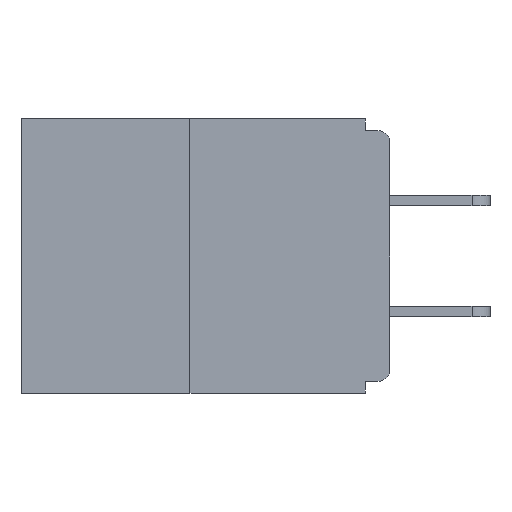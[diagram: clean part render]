
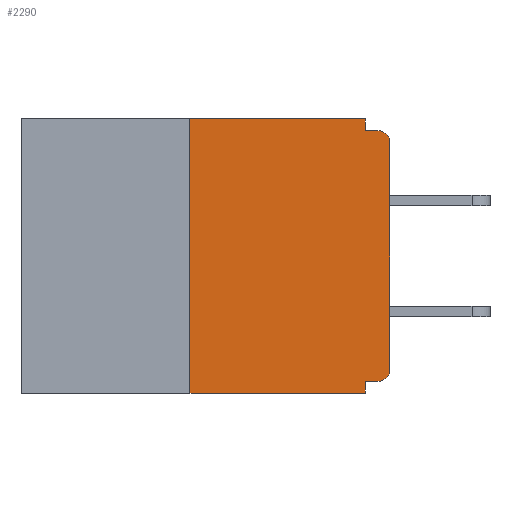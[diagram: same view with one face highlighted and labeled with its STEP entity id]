
A CAD part, left-side view. The second image highlights one B-rep face of the part: STEP entity #2290.
In plain terms, the highlighted planar face has unit normal (-1, 0, 0).
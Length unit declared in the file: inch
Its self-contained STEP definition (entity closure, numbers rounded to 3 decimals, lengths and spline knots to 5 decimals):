
#183 = PLANE ( 'NONE',  #4799 ) ;
#190 = VERTEX_POINT ( 'NONE', #14920 ) ;
#453 = ORIENTED_EDGE ( 'NONE', *, *, #7173, .F. ) ;
#699 = EDGE_CURVE ( 'NONE', #190, #17312, #8416, .T. ) ;
#786 = CARTESIAN_POINT ( 'NONE',  ( 0., 0., -0.03 ) ) ;
#973 = CARTESIAN_POINT ( 'NONE',  ( 0., 0.015, -0.328 ) ) ;
#1226 = VERTEX_POINT ( 'NONE', #10289 ) ;
#1649 = EDGE_CURVE ( 'NONE', #17980, #9314, #11730, .T. ) ;
#1697 = DIRECTION ( 'NONE',  ( 0., 0., -1. ) ) ;
#1724 = CARTESIAN_POINT ( 'NONE',  ( 0., 0., -0.015 ) ) ;
#2184 = CARTESIAN_POINT ( 'NONE',  ( 0., 0.015, -0.313 ) ) ;
#2290 = ADVANCED_FACE ( 'NONE', ( #3118 ), #183, .F. ) ;
#2786 = CARTESIAN_POINT ( 'NONE',  ( 0., 0.46, 0. ) ) ;
#2792 = LINE ( 'NONE', #15246, #10029 ) ;
#2833 = DIRECTION ( 'NONE',  ( 0., 0., 1. ) ) ;
#3118 = FACE_OUTER_BOUND ( 'NONE', #16494, .T. ) ;
#3314 = CARTESIAN_POINT ( 'NONE',  ( 0., 0.031, -0.328 ) ) ;
#3999 = CIRCLE ( 'NONE', #13432, 0.015 ) ;
#4441 = DIRECTION ( 'NONE',  ( 0., 0., -1. ) ) ;
#4478 = DIRECTION ( 'NONE',  ( 1., 0., 0. ) ) ;
#4491 = VERTEX_POINT ( 'NONE', #16919 ) ;
#4651 = EDGE_CURVE ( 'NONE', #17312, #1226, #11841, .T. ) ;
#4799 = AXIS2_PLACEMENT_3D ( 'NONE', #5992, #4478, #1697 ) ;
#4962 = DIRECTION ( 'NONE',  ( 0., 0., -1. ) ) ;
#5008 = ORIENTED_EDGE ( 'NONE', *, *, #4651, .F. ) ;
#5094 = DIRECTION ( 'NONE',  ( 0., 0., -1. ) ) ;
#5135 = CARTESIAN_POINT ( 'NONE',  ( 0., 0.46, -0.343 ) ) ;
#5992 = CARTESIAN_POINT ( 'NONE',  ( 0., 0.46, 0. ) ) ;
#6024 = DIRECTION ( 'NONE',  ( 0., -1., 0. ) ) ;
#7113 = VERTEX_POINT ( 'NONE', #15981 ) ;
#7124 = ORIENTED_EDGE ( 'NONE', *, *, #18024, .T. ) ;
#7173 = EDGE_CURVE ( 'NONE', #10045, #7966, #10859, .T. ) ;
#7211 = ORIENTED_EDGE ( 'NONE', *, *, #13579, .F. ) ;
#7966 = VERTEX_POINT ( 'NONE', #3314 ) ;
#8043 = VECTOR ( 'NONE', #14109, 39.37008 ) ;
#8416 = LINE ( 'NONE', #2786, #13779 ) ;
#8475 = ORIENTED_EDGE ( 'NONE', *, *, #1649, .T. ) ;
#8771 = VECTOR ( 'NONE', #2833, 39.37008 ) ;
#8884 = CARTESIAN_POINT ( 'NONE',  ( 0., 0.031, 0. ) ) ;
#9164 = CARTESIAN_POINT ( 'NONE',  ( 0., 0.015, -0.015 ) ) ;
#9314 = VERTEX_POINT ( 'NONE', #9164 ) ;
#9770 = EDGE_CURVE ( 'NONE', #1226, #9314, #11956, .T. ) ;
#9935 = DIRECTION ( 'NONE',  ( 0., -1., 0. ) ) ;
#10029 = VECTOR ( 'NONE', #5094, 39.37008 ) ;
#10038 = LINE ( 'NONE', #5135, #8043 ) ;
#10045 = VERTEX_POINT ( 'NONE', #973 ) ;
#10141 = VECTOR ( 'NONE', #13106, 39.37008 ) ;
#10289 = CARTESIAN_POINT ( 'NONE',  ( 0., 0.031, -0.015 ) ) ;
#10817 = DIRECTION ( 'NONE',  ( -1., 0., 0. ) ) ;
#10859 = LINE ( 'NONE', #15917, #11521 ) ;
#11047 = AXIS2_PLACEMENT_3D ( 'NONE', #14009, #10817, #4962 ) ;
#11521 = VECTOR ( 'NONE', #14372, 39.37008 ) ;
#11730 = CIRCLE ( 'NONE', #11047, 0.015 ) ;
#11841 = LINE ( 'NONE', #8884, #16958 ) ;
#11940 = LINE ( 'NONE', #14514, #10141 ) ;
#11956 = LINE ( 'NONE', #1724, #12179 ) ;
#12179 = VECTOR ( 'NONE', #6024, 39.37008 ) ;
#12334 = VERTEX_POINT ( 'NONE', #12442 ) ;
#12442 = CARTESIAN_POINT ( 'NONE',  ( 0., 0., -0.313 ) ) ;
#12531 = EDGE_CURVE ( 'NONE', #7113, #4491, #10038, .T. ) ;
#13106 = DIRECTION ( 'NONE',  ( 0., 0., 1. ) ) ;
#13432 = AXIS2_PLACEMENT_3D ( 'NONE', #2184, #17759, #13663 ) ;
#13579 = EDGE_CURVE ( 'NONE', #7966, #4491, #2792, .T. ) ;
#13663 = DIRECTION ( 'NONE',  ( 0., 0., -1. ) ) ;
#13665 = ORIENTED_EDGE ( 'NONE', *, *, #699, .F. ) ;
#13779 = VECTOR ( 'NONE', #9935, 39.37008 ) ;
#14009 = CARTESIAN_POINT ( 'NONE',  ( 0., 0.015, -0.03 ) ) ;
#14073 = ORIENTED_EDGE ( 'NONE', *, *, #17715, .F. ) ;
#14109 = DIRECTION ( 'NONE',  ( 0., -1., 0. ) ) ;
#14335 = LINE ( 'NONE', #17214, #8771 ) ;
#14372 = DIRECTION ( 'NONE',  ( 0., 1., 0. ) ) ;
#14514 = CARTESIAN_POINT ( 'NONE',  ( 0., 0., 0. ) ) ;
#14787 = ORIENTED_EDGE ( 'NONE', *, *, #12531, .T. ) ;
#14920 = CARTESIAN_POINT ( 'NONE',  ( 0., 0.25, 0. ) ) ;
#15246 = CARTESIAN_POINT ( 'NONE',  ( 0., 0.031, -0.343 ) ) ;
#15334 = ORIENTED_EDGE ( 'NONE', *, *, #16476, .T. ) ;
#15917 = CARTESIAN_POINT ( 'NONE',  ( 0., 0., -0.328 ) ) ;
#15981 = CARTESIAN_POINT ( 'NONE',  ( 0., 0.25, -0.343 ) ) ;
#16476 = EDGE_CURVE ( 'NONE', #12334, #17980, #11940, .T. ) ;
#16494 = EDGE_LOOP ( 'NONE', ( #13665, #14073, #14787, #7211, #453, #7124, #15334, #8475, #17821, #5008 ) ) ;
#16919 = CARTESIAN_POINT ( 'NONE',  ( 0., 0.031, -0.343 ) ) ;
#16958 = VECTOR ( 'NONE', #4441, 39.37008 ) ;
#17119 = CARTESIAN_POINT ( 'NONE',  ( 0., 0.031, 0. ) ) ;
#17214 = CARTESIAN_POINT ( 'NONE',  ( 0., 0.25, 0. ) ) ;
#17312 = VERTEX_POINT ( 'NONE', #17119 ) ;
#17715 = EDGE_CURVE ( 'NONE', #7113, #190, #14335, .T. ) ;
#17759 = DIRECTION ( 'NONE',  ( -1., 0., 0. ) ) ;
#17821 = ORIENTED_EDGE ( 'NONE', *, *, #9770, .F. ) ;
#17980 = VERTEX_POINT ( 'NONE', #786 ) ;
#18024 = EDGE_CURVE ( 'NONE', #10045, #12334, #3999, .T. ) ;
